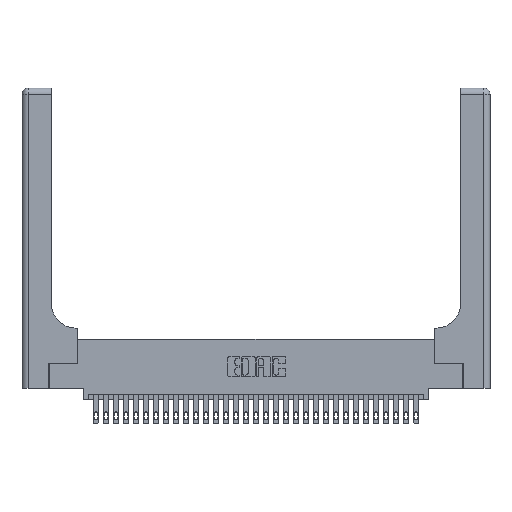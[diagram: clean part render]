
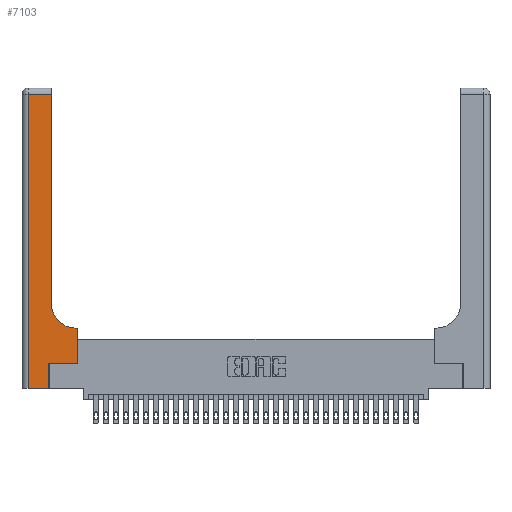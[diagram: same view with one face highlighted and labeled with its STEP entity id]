
A CAD part, top view. The second image highlights one B-rep face of the part: STEP entity #7103.
In plain terms, the highlighted planar face has unit normal (0, 0, 1).
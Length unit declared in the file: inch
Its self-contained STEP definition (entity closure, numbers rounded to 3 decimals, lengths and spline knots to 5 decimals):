
#50 = VERTEX_POINT ( 'NONE', #20989 ) ;
#196 = EDGE_CURVE ( 'NONE', #29774, #7957, #18709, .T. ) ;
#512 = LINE ( 'NONE', #27184, #8403 ) ;
#811 = EDGE_CURVE ( 'NONE', #50, #12405, #24875, .T. ) ;
#1682 = CARTESIAN_POINT ( 'NONE',  ( 0.5415, 0.85, 0.37 ) ) ;
#2377 = LINE ( 'NONE', #13596, #4733 ) ;
#2939 = DIRECTION ( 'NONE',  ( 0., 1., 0. ) ) ;
#3056 = CIRCLE ( 'NONE', #17530, 0.25 ) ;
#3166 = CARTESIAN_POINT ( 'NONE',  ( 0.269, 0.25, 0.37 ) ) ;
#3884 = CARTESIAN_POINT ( 'NONE',  ( 0.06, 3., 0.37 ) ) ;
#4374 = DIRECTION ( 'NONE',  ( -1., 0., 0. ) ) ;
#4422 = LINE ( 'NONE', #18676, #23575 ) ;
#4733 = VECTOR ( 'NONE', #11833, 39.37008 ) ;
#4928 = VECTOR ( 'NONE', #20362, 39.37008 ) ;
#5024 = DIRECTION ( 'NONE',  ( 1., 0., 0. ) ) ;
#5270 = CARTESIAN_POINT ( 'NONE',  ( 0., 2.94, 0.37 ) ) ;
#5542 = ORIENTED_EDGE ( 'NONE', *, *, #6608, .T. ) ;
#5759 = LINE ( 'NONE', #5270, #31514 ) ;
#6608 = EDGE_CURVE ( 'NONE', #10144, #27712, #24529, .T. ) ;
#6841 = CARTESIAN_POINT ( 'NONE',  ( 0., 3., 0.37 ) ) ;
#6874 = ORIENTED_EDGE ( 'NONE', *, *, #811, .T. ) ;
#7103 = ADVANCED_FACE ( 'NONE', ( #32361 ), #23892, .F. ) ;
#7279 = VECTOR ( 'NONE', #4374, 39.37008 ) ;
#7957 = VERTEX_POINT ( 'NONE', #13857 ) ;
#8090 = LINE ( 'NONE', #31743, #7279 ) ;
#8403 = VECTOR ( 'NONE', #5024, 39.37008 ) ;
#8455 = CARTESIAN_POINT ( 'NONE',  ( 0.5585, 0.6, 0.37 ) ) ;
#9899 = DIRECTION ( 'NONE',  ( -1., 0., 0. ) ) ;
#10144 = VERTEX_POINT ( 'NONE', #14269 ) ;
#10543 = CARTESIAN_POINT ( 'NONE',  ( 0.2915, 2.94, 0.37 ) ) ;
#10768 = ORIENTED_EDGE ( 'NONE', *, *, #28478, .T. ) ;
#11833 = DIRECTION ( 'NONE',  ( 1., 0., 0. ) ) ;
#12405 = VERTEX_POINT ( 'NONE', #10543 ) ;
#13076 = VERTEX_POINT ( 'NONE', #31315 ) ;
#13596 = CARTESIAN_POINT ( 'NONE',  ( 0., 0., 0.37 ) ) ;
#13857 = CARTESIAN_POINT ( 'NONE',  ( 0.06, 0., 0.37 ) ) ;
#14269 = CARTESIAN_POINT ( 'NONE',  ( 0.269, 0., 0.37 ) ) ;
#16067 = EDGE_LOOP ( 'NONE', ( #6874, #18362, #25377, #25407, #5542, #22042, #18140, #31073, #10768 ) ) ;
#16495 = DIRECTION ( 'NONE',  ( 0., 0., -1. ) ) ;
#16731 = DIRECTION ( 'NONE',  ( 0., 0., -1. ) ) ;
#17251 = VECTOR ( 'NONE', #2939, 39.37008 ) ;
#17325 = VERTEX_POINT ( 'NONE', #8455 ) ;
#17530 = AXIS2_PLACEMENT_3D ( 'NONE', #1682, #16731, #23785 ) ;
#17606 = CARTESIAN_POINT ( 'NONE',  ( 0.5585, 0.25, 0.37 ) ) ;
#18140 = ORIENTED_EDGE ( 'NONE', *, *, #25250, .T. ) ;
#18285 = CARTESIAN_POINT ( 'NONE',  ( 0.269, 0., 0.37 ) ) ;
#18362 = ORIENTED_EDGE ( 'NONE', *, *, #20101, .T. ) ;
#18676 = CARTESIAN_POINT ( 'NONE',  ( 0.5585, 0.25, 0.37 ) ) ;
#18693 = DIRECTION ( 'NONE',  ( 0., -1., 0. ) ) ;
#18709 = LINE ( 'NONE', #3884, #19476 ) ;
#19476 = VECTOR ( 'NONE', #18693, 39.37008 ) ;
#20046 = CARTESIAN_POINT ( 'NONE',  ( 0.2915, 3., 0.37 ) ) ;
#20101 = EDGE_CURVE ( 'NONE', #12405, #29774, #5759, .T. ) ;
#20362 = DIRECTION ( 'NONE',  ( 0., 1., 0. ) ) ;
#20503 = EDGE_CURVE ( 'NONE', #17325, #13076, #8090, .T. ) ;
#20989 = CARTESIAN_POINT ( 'NONE',  ( 0.2915, 0.85, 0.37 ) ) ;
#21792 = EDGE_CURVE ( 'NONE', #27712, #24977, #512, .T. ) ;
#22042 = ORIENTED_EDGE ( 'NONE', *, *, #21792, .T. ) ;
#22988 = EDGE_CURVE ( 'NONE', #7957, #10144, #2377, .T. ) ;
#23575 = VECTOR ( 'NONE', #31246, 39.37008 ) ;
#23785 = DIRECTION ( 'NONE',  ( 1., 0., 0. ) ) ;
#23892 = PLANE ( 'NONE',  #30968 ) ;
#24529 = LINE ( 'NONE', #18285, #17251 ) ;
#24875 = LINE ( 'NONE', #20046, #4928 ) ;
#24977 = VERTEX_POINT ( 'NONE', #17606 ) ;
#25250 = EDGE_CURVE ( 'NONE', #24977, #17325, #4422, .T. ) ;
#25377 = ORIENTED_EDGE ( 'NONE', *, *, #196, .T. ) ;
#25407 = ORIENTED_EDGE ( 'NONE', *, *, #22988, .T. ) ;
#26489 = DIRECTION ( 'NONE',  ( -1., 0., 0. ) ) ;
#27184 = CARTESIAN_POINT ( 'NONE',  ( 0.269, 0.25, 0.37 ) ) ;
#27712 = VERTEX_POINT ( 'NONE', #3166 ) ;
#28478 = EDGE_CURVE ( 'NONE', #13076, #50, #3056, .T. ) ;
#29774 = VERTEX_POINT ( 'NONE', #30977 ) ;
#30968 = AXIS2_PLACEMENT_3D ( 'NONE', #6841, #16495, #26489 ) ;
#30977 = CARTESIAN_POINT ( 'NONE',  ( 0.06, 2.94, 0.37 ) ) ;
#31073 = ORIENTED_EDGE ( 'NONE', *, *, #20503, .T. ) ;
#31246 = DIRECTION ( 'NONE',  ( 0., 1., 0. ) ) ;
#31315 = CARTESIAN_POINT ( 'NONE',  ( 0.5415, 0.6, 0.37 ) ) ;
#31514 = VECTOR ( 'NONE', #9899, 39.37008 ) ;
#31743 = CARTESIAN_POINT ( 'NONE',  ( 0.2915, 0.6, 0.37 ) ) ;
#32361 = FACE_OUTER_BOUND ( 'NONE', #16067, .T. ) ;
